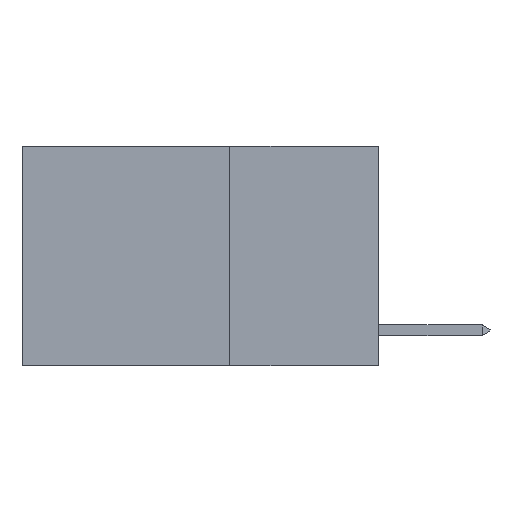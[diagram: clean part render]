
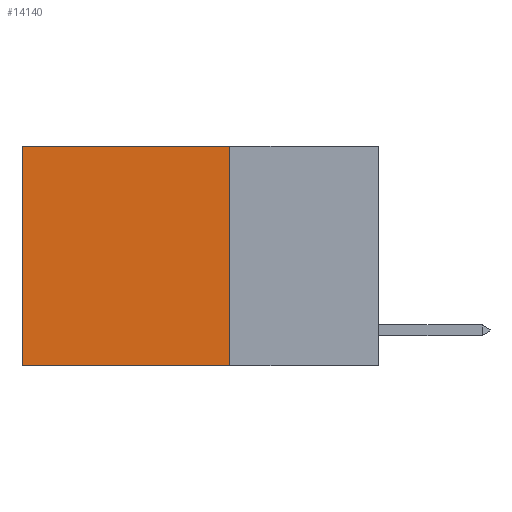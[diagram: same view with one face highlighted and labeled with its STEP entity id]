
A CAD part, left-side view. The second image highlights one B-rep face of the part: STEP entity #14140.
In plain terms, the highlighted planar face has unit normal (-1, 0, 0).
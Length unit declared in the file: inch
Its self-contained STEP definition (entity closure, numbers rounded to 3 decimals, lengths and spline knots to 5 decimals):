
#917 = AXIS2_PLACEMENT_3D ( 'NONE', #19451, #16252, #6191 ) ;
#1829 = LINE ( 'NONE', #14680, #10973 ) ;
#1888 = VERTEX_POINT ( 'NONE', #14402 ) ;
#3116 = ORIENTED_EDGE ( 'NONE', *, *, #17009, .F. ) ;
#4533 = DIRECTION ( 'NONE',  ( 0., 0., -1. ) ) ;
#4834 = LINE ( 'NONE', #10327, #21479 ) ;
#6191 = DIRECTION ( 'NONE',  ( 0., 0., -1. ) ) ;
#7341 = VECTOR ( 'NONE', #17727, 39.37008 ) ;
#9137 = LINE ( 'NONE', #19250, #17489 ) ;
#9317 = ORIENTED_EDGE ( 'NONE', *, *, #16066, .F. ) ;
#9656 = EDGE_LOOP ( 'NONE', ( #18297, #3116, #9317, #10990 ) ) ;
#10327 = CARTESIAN_POINT ( 'NONE',  ( 0.2625, 0.25, -0.37 ) ) ;
#10973 = VECTOR ( 'NONE', #4533, 39.37008 ) ;
#10990 = ORIENTED_EDGE ( 'NONE', *, *, #21555, .T. ) ;
#11836 = LINE ( 'NONE', #12786, #7341 ) ;
#12392 = CARTESIAN_POINT ( 'NONE',  ( 0.2625, 0.6, -0.37 ) ) ;
#12409 = CARTESIAN_POINT ( 'NONE',  ( 0.2625, 0.25, 0. ) ) ;
#12768 = VERTEX_POINT ( 'NONE', #12392 ) ;
#12786 = CARTESIAN_POINT ( 'NONE',  ( 0.2625, 0.6, 0. ) ) ;
#12847 = CARTESIAN_POINT ( 'NONE',  ( 0.2625, 0.6, 0. ) ) ;
#14140 = ADVANCED_FACE ( 'NONE', ( #19341 ), #21088, .F. ) ;
#14402 = CARTESIAN_POINT ( 'NONE',  ( 0.2625, 0.25, -0.37 ) ) ;
#14680 = CARTESIAN_POINT ( 'NONE',  ( 0.2625, 0.25, 0. ) ) ;
#14744 = EDGE_CURVE ( 'NONE', #16674, #12768, #11836, .T. ) ;
#16066 = EDGE_CURVE ( 'NONE', #17802, #1888, #1829, .T. ) ;
#16252 = DIRECTION ( 'NONE',  ( 1., 0., 0. ) ) ;
#16674 = VERTEX_POINT ( 'NONE', #12847 ) ;
#17009 = EDGE_CURVE ( 'NONE', #1888, #12768, #4834, .T. ) ;
#17489 = VECTOR ( 'NONE', #20903, 39.37008 ) ;
#17727 = DIRECTION ( 'NONE',  ( 0., 0., -1. ) ) ;
#17802 = VERTEX_POINT ( 'NONE', #12409 ) ;
#18297 = ORIENTED_EDGE ( 'NONE', *, *, #14744, .T. ) ;
#18605 = DIRECTION ( 'NONE',  ( 0., 1., 0. ) ) ;
#19250 = CARTESIAN_POINT ( 'NONE',  ( 0.2625, 0.25, 0. ) ) ;
#19341 = FACE_OUTER_BOUND ( 'NONE', #9656, .T. ) ;
#19451 = CARTESIAN_POINT ( 'NONE',  ( 0.2625, 0.25, 0. ) ) ;
#20903 = DIRECTION ( 'NONE',  ( 0., 1., 0. ) ) ;
#21088 = PLANE ( 'NONE',  #917 ) ;
#21479 = VECTOR ( 'NONE', #18605, 39.37008 ) ;
#21555 = EDGE_CURVE ( 'NONE', #17802, #16674, #9137, .T. ) ;
